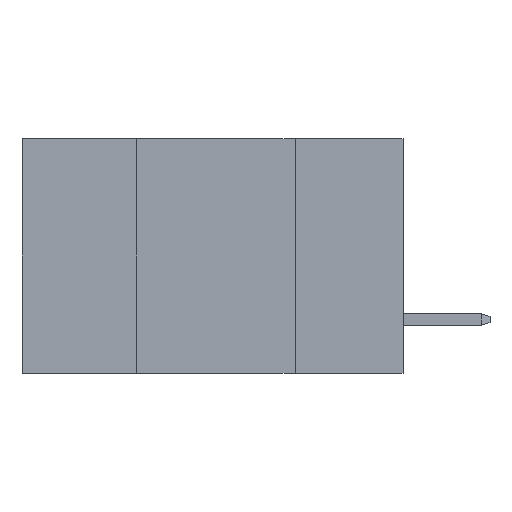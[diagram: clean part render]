
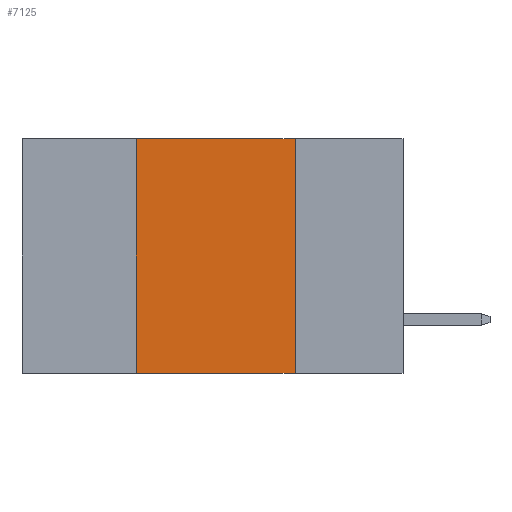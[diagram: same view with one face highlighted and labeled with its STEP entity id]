
A CAD part, left-side view. The second image highlights one B-rep face of the part: STEP entity #7125.
In plain terms, the highlighted planar face has unit normal (-1, 0, 0).
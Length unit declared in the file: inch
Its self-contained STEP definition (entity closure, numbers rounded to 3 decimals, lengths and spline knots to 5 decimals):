
#37 = ORIENTED_EDGE ( 'NONE', *, *, #5996, .F. ) ;
#394 = CARTESIAN_POINT ( 'NONE',  ( 0., 0.6, -0.37 ) ) ;
#455 = LINE ( 'NONE', #394, #10226 ) ;
#645 = CARTESIAN_POINT ( 'NONE',  ( 0., 0.17, -0.37 ) ) ;
#806 = ORIENTED_EDGE ( 'NONE', *, *, #7880, .F. ) ;
#1226 = VECTOR ( 'NONE', #2429, 39.37008 ) ;
#1373 = VERTEX_POINT ( 'NONE', #4072 ) ;
#2429 = DIRECTION ( 'NONE',  ( 0., 0., -1. ) ) ;
#3509 = LINE ( 'NONE', #5340, #11985 ) ;
#4072 = CARTESIAN_POINT ( 'NONE',  ( 0., 0.42, -0.37 ) ) ;
#4133 = CARTESIAN_POINT ( 'NONE',  ( 0., 0.42, 0. ) ) ;
#4352 = DIRECTION ( 'NONE',  ( 1., 0., 0. ) ) ;
#4548 = LINE ( 'NONE', #8833, #1226 ) ;
#4670 = DIRECTION ( 'NONE',  ( 0., -1., 0. ) ) ;
#5183 = EDGE_CURVE ( 'NONE', #1373, #7411, #455, .T. ) ;
#5340 = CARTESIAN_POINT ( 'NONE',  ( 0., 0.42, 0. ) ) ;
#5891 = CARTESIAN_POINT ( 'NONE',  ( 0., 0.17, 0. ) ) ;
#5996 = EDGE_CURVE ( 'NONE', #12275, #7411, #4548, .T. ) ;
#6653 = EDGE_LOOP ( 'NONE', ( #37, #806, #8027, #11871 ) ) ;
#7125 = ADVANCED_FACE ( 'NONE', ( #9493 ), #12687, .F. ) ;
#7411 = VERTEX_POINT ( 'NONE', #645 ) ;
#7880 = EDGE_CURVE ( 'NONE', #13841, #12275, #8193, .T. ) ;
#8027 = ORIENTED_EDGE ( 'NONE', *, *, #12176, .F. ) ;
#8193 = LINE ( 'NONE', #12503, #9541 ) ;
#8833 = CARTESIAN_POINT ( 'NONE',  ( 0., 0.17, 0. ) ) ;
#9493 = FACE_OUTER_BOUND ( 'NONE', #6653, .T. ) ;
#9541 = VECTOR ( 'NONE', #13480, 39.37008 ) ;
#9627 = DIRECTION ( 'NONE',  ( 0., 0., 1. ) ) ;
#10212 = AXIS2_PLACEMENT_3D ( 'NONE', #10698, #4352, #10504 ) ;
#10226 = VECTOR ( 'NONE', #4670, 39.37008 ) ;
#10504 = DIRECTION ( 'NONE',  ( 0., 0., -1. ) ) ;
#10698 = CARTESIAN_POINT ( 'NONE',  ( 0., 0.6, 0. ) ) ;
#11871 = ORIENTED_EDGE ( 'NONE', *, *, #5183, .T. ) ;
#11985 = VECTOR ( 'NONE', #9627, 39.37008 ) ;
#12176 = EDGE_CURVE ( 'NONE', #1373, #13841, #3509, .T. ) ;
#12275 = VERTEX_POINT ( 'NONE', #5891 ) ;
#12503 = CARTESIAN_POINT ( 'NONE',  ( 0., 0.6, 0. ) ) ;
#12687 = PLANE ( 'NONE',  #10212 ) ;
#13480 = DIRECTION ( 'NONE',  ( 0., -1., 0. ) ) ;
#13841 = VERTEX_POINT ( 'NONE', #4133 ) ;
